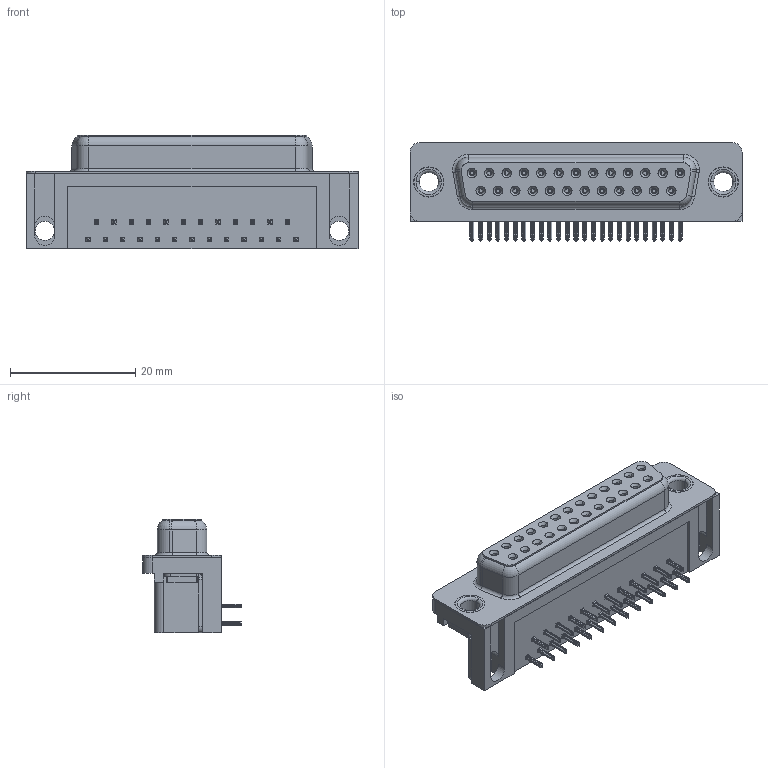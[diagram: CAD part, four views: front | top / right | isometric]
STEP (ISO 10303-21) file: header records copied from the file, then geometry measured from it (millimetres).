
FILE_DESCRIPTION (( 'STEP AP203' ), '1' );
FILE_NAME ('622-025-668-011.STEP', '2019-11-20T05:05:54', ( '' ), ( '' ), 'SwSTEP 2.0', 'SolidWorks 2016', '' );
FILE_SCHEMA (( 'CONFIG_CONTROL_DESIGN' ));
Length unit declared in the file: millimetre
Products named in the file (7): 622 Thru Hole Board Mount; 622 Contact Top; 622 Socket Bottom; 622-025-668-011; 622 Housing_25 Socket; 622 Shell_25 Socket; 622 Thru Hole Rivet
Assembly tree (31 placements, depth 2):
  622-025-668-011
    622 Housing_25 Socket
    622 Shell_25 Socket
    622 Socket Bottom  x12
    622 Contact Top  x13
    622 Thru Hole Board Mount  x2
    622 Thru Hole Rivet  x2
Bounding box: 53.04 x 15.73 x 18.2 mm (x, y, z)
Volume: 7588.6 mm3; surface area: 9404.3 mm2
Topology: 31 solids, 31 shells, 3810 faces, 9992 edges, 6264 vertices
Faces by surface type: plane 1722, cylinder 902, bspline 852, cone 300, torus 34
Entity records: 28644 total; most frequent: CARTESIAN_POINT 7846, ORIENTED_EDGE 4100, DIRECTION 3810, EDGE_CURVE 2050, LINE 1352, VECTOR 1352, VERTEX_POINT 1308, AXIS2_PLACEMENT_3D 1229
